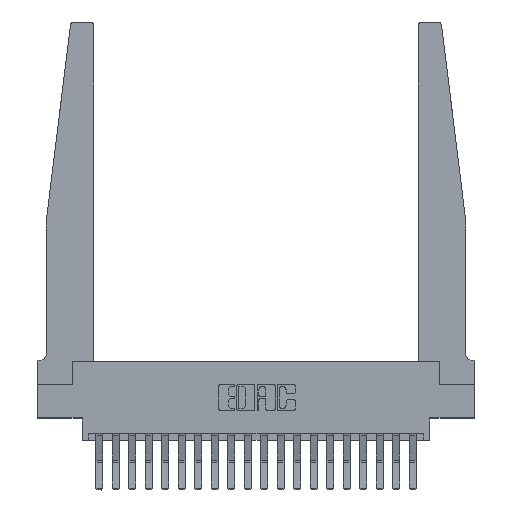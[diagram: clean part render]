
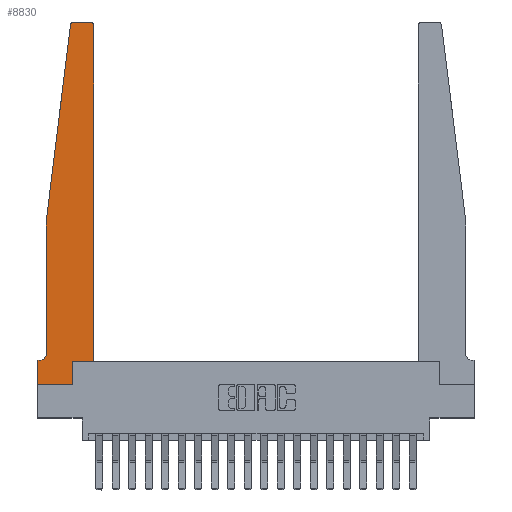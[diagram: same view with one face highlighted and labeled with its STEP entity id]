
A CAD part, top view. The second image highlights one B-rep face of the part: STEP entity #8830.
In plain terms, the highlighted planar face has unit normal (0, 0, 1).
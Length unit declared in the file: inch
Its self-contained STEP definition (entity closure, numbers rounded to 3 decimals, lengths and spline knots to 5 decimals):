
#9 = VERTEX_POINT ( 'NONE', #5638 ) ;
#51 = CIRCLE ( 'NONE', #7845, 0.05 ) ;
#506 = CARTESIAN_POINT ( 'NONE',  ( 0.065, 1.25, 0.37 ) ) ;
#817 = CARTESIAN_POINT ( 'NONE',  ( 0.065, 1.25, 0.37 ) ) ;
#1069 = VERTEX_POINT ( 'NONE', #12058 ) ;
#1137 = DIRECTION ( 'NONE',  ( 0., 0., -1. ) ) ;
#1458 = CARTESIAN_POINT ( 'NONE',  ( 0., 0., 0.37 ) ) ;
#1721 = DIRECTION ( 'NONE',  ( 0., -1., 0. ) ) ;
#2143 = CARTESIAN_POINT ( 'NONE',  ( 0., 0.1875, 0.37 ) ) ;
#2310 = DIRECTION ( 'NONE',  ( -1., 0., 0. ) ) ;
#2396 = EDGE_CURVE ( 'NONE', #7685, #16128, #51, .T. ) ;
#2440 = LINE ( 'NONE', #20093, #19192 ) ;
#2795 = EDGE_CURVE ( 'NONE', #4970, #9732, #18815, .T. ) ;
#3255 = EDGE_CURVE ( 'NONE', #9732, #7685, #10127, .T. ) ;
#4204 = ORIENTED_EDGE ( 'NONE', *, *, #2795, .T. ) ;
#4298 = CARTESIAN_POINT ( 'NONE',  ( 0., 0., 0.37 ) ) ;
#4970 = VERTEX_POINT ( 'NONE', #18944 ) ;
#5011 = EDGE_CURVE ( 'NONE', #20192, #15367, #15410, .T. ) ;
#5033 = DIRECTION ( 'NONE',  ( 0., 1., 0. ) ) ;
#5516 = LINE ( 'NONE', #6910, #17423 ) ;
#5638 = CARTESIAN_POINT ( 'NONE',  ( 0.2605, 0., 0.37 ) ) ;
#5832 = DIRECTION ( 'NONE',  ( 0., 0., 1. ) ) ;
#5836 = VECTOR ( 'NONE', #1721, 39.37008 ) ;
#6095 = LINE ( 'NONE', #18008, #9875 ) ;
#6371 = VECTOR ( 'NONE', #15353, 39.37008 ) ;
#6910 = CARTESIAN_POINT ( 'NONE',  ( 0., 0., 0.37 ) ) ;
#7086 = DIRECTION ( 'NONE',  ( 1., 0., 0. ) ) ;
#7235 = ORIENTED_EDGE ( 'NONE', *, *, #2396, .T. ) ;
#7255 = ORIENTED_EDGE ( 'NONE', *, *, #19818, .T. ) ;
#7337 = CARTESIAN_POINT ( 'NONE',  ( 0.395, 2.72, 0.37 ) ) ;
#7373 = FACE_OUTER_BOUND ( 'NONE', #18165, .T. ) ;
#7479 = EDGE_CURVE ( 'NONE', #16128, #15342, #9951, .T. ) ;
#7500 = PLANE ( 'NONE',  #18043 ) ;
#7676 = CARTESIAN_POINT ( 'NONE',  ( 0.425, 0.18, 0.37 ) ) ;
#7685 = VERTEX_POINT ( 'NONE', #20081 ) ;
#7845 = AXIS2_PLACEMENT_3D ( 'NONE', #10779, #1137, #12444 ) ;
#8029 = ORIENTED_EDGE ( 'NONE', *, *, #12128, .T. ) ;
#8100 = CARTESIAN_POINT ( 'NONE',  ( 0.065, 1.25, 0.37 ) ) ;
#8628 = EDGE_CURVE ( 'NONE', #16630, #20192, #14797, .T. ) ;
#8691 = CARTESIAN_POINT ( 'NONE',  ( 0.27653, 2.75, 0.37 ) ) ;
#8702 = ORIENTED_EDGE ( 'NONE', *, *, #19637, .T. ) ;
#8830 = ADVANCED_FACE ( 'NONE', ( #7373 ), #7500, .T. ) ;
#8966 = DIRECTION ( 'NONE',  ( 1., 0., 0. ) ) ;
#9132 = DIRECTION ( 'NONE',  ( 0., 0., 1. ) ) ;
#9732 = VERTEX_POINT ( 'NONE', #506 ) ;
#9778 = ORIENTED_EDGE ( 'NONE', *, *, #5011, .T. ) ;
#9875 = VECTOR ( 'NONE', #5033, 39.37008 ) ;
#9951 = LINE ( 'NONE', #11112, #13794 ) ;
#10079 = EDGE_CURVE ( 'NONE', #9, #16630, #6095, .T. ) ;
#10084 = CARTESIAN_POINT ( 'NONE',  ( 0.425, 0.18, 0.37 ) ) ;
#10127 = LINE ( 'NONE', #8100, #5836 ) ;
#10779 = CARTESIAN_POINT ( 'NONE',  ( 0.015, 0.2375, 0.37 ) ) ;
#11067 = VECTOR ( 'NONE', #20697, 39.37008 ) ;
#11112 = CARTESIAN_POINT ( 'NONE',  ( 0.065, 0.1875, 0.37 ) ) ;
#11605 = EDGE_CURVE ( 'NONE', #15367, #1069, #13654, .T. ) ;
#11801 = DIRECTION ( 'NONE',  ( 1., 0., 0. ) ) ;
#11835 = ORIENTED_EDGE ( 'NONE', *, *, #8628, .T. ) ;
#12058 = CARTESIAN_POINT ( 'NONE',  ( 0.395, 2.75, 0.37 ) ) ;
#12128 = EDGE_CURVE ( 'NONE', #13024, #9, #5516, .T. ) ;
#12444 = DIRECTION ( 'NONE',  ( -1., 0., 0. ) ) ;
#12540 = ORIENTED_EDGE ( 'NONE', *, *, #21019, .T. ) ;
#13024 = VERTEX_POINT ( 'NONE', #4298 ) ;
#13654 = CIRCLE ( 'NONE', #19164, 0.03 ) ;
#13794 = VECTOR ( 'NONE', #20867, 39.37008 ) ;
#14174 = ORIENTED_EDGE ( 'NONE', *, *, #11605, .T. ) ;
#14660 = VECTOR ( 'NONE', #19328, 39.37008 ) ;
#14797 = LINE ( 'NONE', #16851, #19123 ) ;
#15342 = VERTEX_POINT ( 'NONE', #2143 ) ;
#15353 = DIRECTION ( 'NONE',  ( -0.122, -0.992, 0. ) ) ;
#15367 = VERTEX_POINT ( 'NONE', #16807 ) ;
#15410 = LINE ( 'NONE', #7676, #11067 ) ;
#15554 = CARTESIAN_POINT ( 'NONE',  ( 0.27653, 2.72, 0.37 ) ) ;
#16125 = ORIENTED_EDGE ( 'NONE', *, *, #10079, .T. ) ;
#16128 = VERTEX_POINT ( 'NONE', #18704 ) ;
#16354 = ORIENTED_EDGE ( 'NONE', *, *, #7479, .T. ) ;
#16618 = ORIENTED_EDGE ( 'NONE', *, *, #3255, .T. ) ;
#16630 = VERTEX_POINT ( 'NONE', #19959 ) ;
#16632 = VERTEX_POINT ( 'NONE', #8691 ) ;
#16807 = CARTESIAN_POINT ( 'NONE',  ( 0.425, 2.72, 0.37 ) ) ;
#16851 = CARTESIAN_POINT ( 'NONE',  ( 0.425, 0.18, 0.37 ) ) ;
#17172 = DIRECTION ( 'NONE',  ( 1., 0., 0. ) ) ;
#17423 = VECTOR ( 'NONE', #11801, 39.37008 ) ;
#18008 = CARTESIAN_POINT ( 'NONE',  ( 0.2605, 0.18, 0.37 ) ) ;
#18043 = AXIS2_PLACEMENT_3D ( 'NONE', #18915, #9132, #20520 ) ;
#18165 = EDGE_LOOP ( 'NONE', ( #12540, #8702, #4204, #16618, #7235, #16354, #7255, #8029, #16125, #11835, #9778, #14174 ) ) ;
#18704 = CARTESIAN_POINT ( 'NONE',  ( 0.015, 0.1875, 0.37 ) ) ;
#18745 = DIRECTION ( 'NONE',  ( 0., 0., 1. ) ) ;
#18815 = LINE ( 'NONE', #817, #6371 ) ;
#18915 = CARTESIAN_POINT ( 'NONE',  ( 0., 0.1875, 0.37 ) ) ;
#18944 = CARTESIAN_POINT ( 'NONE',  ( 0.24675, 2.72367, 0.37 ) ) ;
#19123 = VECTOR ( 'NONE', #7086, 39.37008 ) ;
#19164 = AXIS2_PLACEMENT_3D ( 'NONE', #7337, #18745, #8966 ) ;
#19192 = VECTOR ( 'NONE', #2310, 39.37008 ) ;
#19328 = DIRECTION ( 'NONE',  ( 0., -1., 0. ) ) ;
#19637 = EDGE_CURVE ( 'NONE', #16632, #4970, #20065, .T. ) ;
#19818 = EDGE_CURVE ( 'NONE', #15342, #13024, #19998, .T. ) ;
#19959 = CARTESIAN_POINT ( 'NONE',  ( 0.2605, 0.18, 0.37 ) ) ;
#19998 = LINE ( 'NONE', #1458, #14660 ) ;
#20065 = CIRCLE ( 'NONE', #20968, 0.03 ) ;
#20081 = CARTESIAN_POINT ( 'NONE',  ( 0.065, 0.2375, 0.37 ) ) ;
#20093 = CARTESIAN_POINT ( 'NONE',  ( 0.25, 2.75, 0.37 ) ) ;
#20192 = VERTEX_POINT ( 'NONE', #10084 ) ;
#20520 = DIRECTION ( 'NONE',  ( 1., 0., 0. ) ) ;
#20697 = DIRECTION ( 'NONE',  ( 0., 1., 0. ) ) ;
#20867 = DIRECTION ( 'NONE',  ( -1., 0., 0. ) ) ;
#20968 = AXIS2_PLACEMENT_3D ( 'NONE', #15554, #5832, #17172 ) ;
#21019 = EDGE_CURVE ( 'NONE', #1069, #16632, #2440, .T. ) ;
